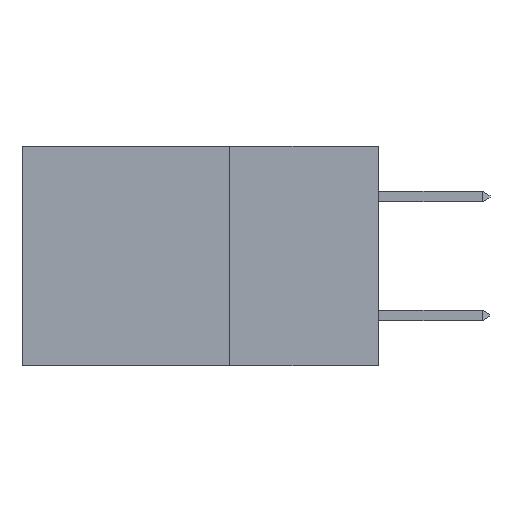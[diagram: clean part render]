
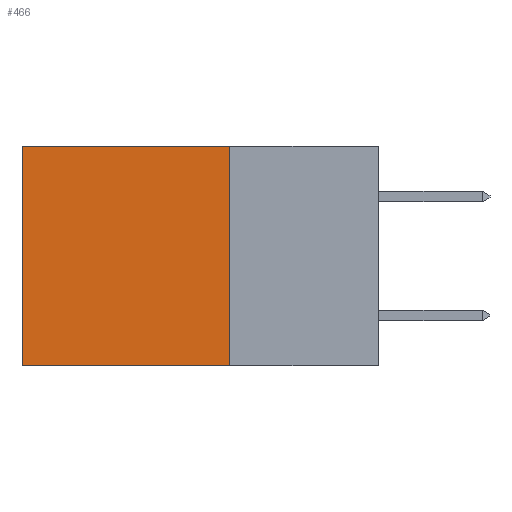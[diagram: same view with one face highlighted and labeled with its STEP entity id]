
A CAD part, left-side view. The second image highlights one B-rep face of the part: STEP entity #466.
In plain terms, the highlighted planar face has unit normal (-1, 0, 0).
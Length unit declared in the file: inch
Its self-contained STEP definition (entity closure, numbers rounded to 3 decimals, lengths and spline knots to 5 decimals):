
#50 = EDGE_CURVE ( 'NONE', #12020, #13052, #6053, .T. ) ;
#52 = FACE_OUTER_BOUND ( 'NONE', #10134, .T. ) ;
#90 = CARTESIAN_POINT ( 'NONE',  ( 0.298, 0.25, 0. ) ) ;
#285 = CARTESIAN_POINT ( 'NONE',  ( 0.298, 0.25, -0.37 ) ) ;
#466 = ADVANCED_FACE ( 'NONE', ( #52 ), #10141, .F. ) ;
#513 = ORIENTED_EDGE ( 'NONE', *, *, #9361, .F. ) ;
#1149 = VECTOR ( 'NONE', #14411, 39.37008 ) ;
#1651 = EDGE_CURVE ( 'NONE', #8665, #12020, #14327, .T. ) ;
#1854 = CARTESIAN_POINT ( 'NONE',  ( 0.298, 0.6, -0.37 ) ) ;
#1875 = ORIENTED_EDGE ( 'NONE', *, *, #1651, .T. ) ;
#2246 = ORIENTED_EDGE ( 'NONE', *, *, #50, .T. ) ;
#2463 = EDGE_CURVE ( 'NONE', #6737, #13052, #8993, .T. ) ;
#3270 = CARTESIAN_POINT ( 'NONE',  ( 0.298, 0.25, 0. ) ) ;
#3709 = ORIENTED_EDGE ( 'NONE', *, *, #2463, .F. ) ;
#5544 = VECTOR ( 'NONE', #15601, 39.37008 ) ;
#6053 = LINE ( 'NONE', #16915, #13348 ) ;
#6737 = VERTEX_POINT ( 'NONE', #285 ) ;
#7400 = VECTOR ( 'NONE', #12752, 39.37008 ) ;
#8249 = LINE ( 'NONE', #13071, #1149 ) ;
#8665 = VERTEX_POINT ( 'NONE', #90 ) ;
#8769 = CARTESIAN_POINT ( 'NONE',  ( 0.298, 0.6, 0. ) ) ;
#8993 = LINE ( 'NONE', #14487, #5544 ) ;
#9361 = EDGE_CURVE ( 'NONE', #8665, #6737, #8249, .T. ) ;
#10031 = DIRECTION ( 'NONE',  ( 0., 0., -1. ) ) ;
#10067 = DIRECTION ( 'NONE',  ( 1., 0., 0. ) ) ;
#10106 = CARTESIAN_POINT ( 'NONE',  ( 0.298, 0.25, 0. ) ) ;
#10134 = EDGE_LOOP ( 'NONE', ( #2246, #3709, #513, #1875 ) ) ;
#10141 = PLANE ( 'NONE',  #14682 ) ;
#12020 = VERTEX_POINT ( 'NONE', #8769 ) ;
#12752 = DIRECTION ( 'NONE',  ( 0., 1., 0. ) ) ;
#13052 = VERTEX_POINT ( 'NONE', #1854 ) ;
#13071 = CARTESIAN_POINT ( 'NONE',  ( 0.298, 0.25, 0. ) ) ;
#13348 = VECTOR ( 'NONE', #16594, 39.37008 ) ;
#14327 = LINE ( 'NONE', #3270, #7400 ) ;
#14411 = DIRECTION ( 'NONE',  ( 0., 0., -1. ) ) ;
#14487 = CARTESIAN_POINT ( 'NONE',  ( 0.298, 0.25, -0.37 ) ) ;
#14682 = AXIS2_PLACEMENT_3D ( 'NONE', #10106, #10067, #10031 ) ;
#15601 = DIRECTION ( 'NONE',  ( 0., 1., 0. ) ) ;
#16594 = DIRECTION ( 'NONE',  ( 0., 0., -1. ) ) ;
#16915 = CARTESIAN_POINT ( 'NONE',  ( 0.298, 0.6, 0. ) ) ;
